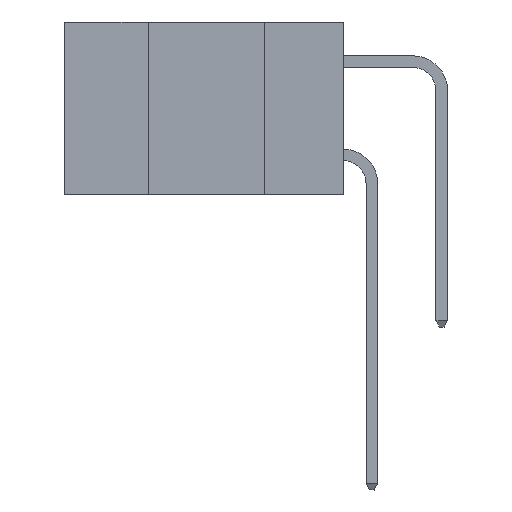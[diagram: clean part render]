
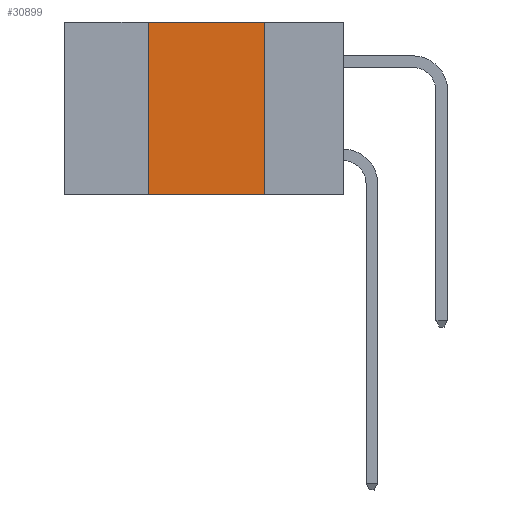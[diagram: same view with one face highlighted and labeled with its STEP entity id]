
A CAD part, left-side view. The second image highlights one B-rep face of the part: STEP entity #30899.
In plain terms, the highlighted planar face has unit normal (-1, 0, 0).
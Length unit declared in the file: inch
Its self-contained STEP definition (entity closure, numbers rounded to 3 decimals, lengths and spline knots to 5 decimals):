
#1603 = CARTESIAN_POINT ( 'NONE',  ( 0., 0.17, 0. ) ) ;
#2638 = LINE ( 'NONE', #18687, #22733 ) ;
#3861 = EDGE_LOOP ( 'NONE', ( #24879, #13345, #13877, #4963 ) ) ;
#4963 = ORIENTED_EDGE ( 'NONE', *, *, #8448, .T. ) ;
#5299 = VERTEX_POINT ( 'NONE', #20327 ) ;
#5952 = CARTESIAN_POINT ( 'NONE',  ( 0., 0.17, -0.37 ) ) ;
#6713 = AXIS2_PLACEMENT_3D ( 'NONE', #21900, #19490, #26617 ) ;
#8412 = DIRECTION ( 'NONE',  ( 0., -1., 0. ) ) ;
#8448 = EDGE_CURVE ( 'NONE', #5299, #20768, #2638, .T. ) ;
#8605 = DIRECTION ( 'NONE',  ( 0., 0., 1. ) ) ;
#9638 = FACE_OUTER_BOUND ( 'NONE', #3861, .T. ) ;
#12468 = VECTOR ( 'NONE', #21956, 39.37008 ) ;
#13230 = VERTEX_POINT ( 'NONE', #1603 ) ;
#13345 = ORIENTED_EDGE ( 'NONE', *, *, #16506, .F. ) ;
#13877 = ORIENTED_EDGE ( 'NONE', *, *, #30477, .F. ) ;
#14212 = EDGE_CURVE ( 'NONE', #13230, #20768, #14432, .T. ) ;
#14432 = LINE ( 'NONE', #19221, #12468 ) ;
#14481 = PLANE ( 'NONE',  #6713 ) ;
#15494 = VERTEX_POINT ( 'NONE', #31710 ) ;
#15525 = DIRECTION ( 'NONE',  ( 0., -1., 0. ) ) ;
#16506 = EDGE_CURVE ( 'NONE', #15494, #13230, #30037, .T. ) ;
#18687 = CARTESIAN_POINT ( 'NONE',  ( 0., 0.6, -0.37 ) ) ;
#18761 = CARTESIAN_POINT ( 'NONE',  ( 0., 0.42, 0. ) ) ;
#19221 = CARTESIAN_POINT ( 'NONE',  ( 0., 0.17, 0. ) ) ;
#19490 = DIRECTION ( 'NONE',  ( 1., 0., 0. ) ) ;
#20327 = CARTESIAN_POINT ( 'NONE',  ( 0., 0.42, -0.37 ) ) ;
#20768 = VERTEX_POINT ( 'NONE', #5952 ) ;
#21900 = CARTESIAN_POINT ( 'NONE',  ( 0., 0.6, 0. ) ) ;
#21907 = VECTOR ( 'NONE', #8605, 39.37008 ) ;
#21956 = DIRECTION ( 'NONE',  ( 0., 0., -1. ) ) ;
#22733 = VECTOR ( 'NONE', #8412, 39.37008 ) ;
#23373 = VECTOR ( 'NONE', #15525, 39.37008 ) ;
#24879 = ORIENTED_EDGE ( 'NONE', *, *, #14212, .F. ) ;
#25620 = CARTESIAN_POINT ( 'NONE',  ( 0., 0.6, 0. ) ) ;
#26617 = DIRECTION ( 'NONE',  ( 0., 0., -1. ) ) ;
#28559 = LINE ( 'NONE', #18761, #21907 ) ;
#30037 = LINE ( 'NONE', #25620, #23373 ) ;
#30477 = EDGE_CURVE ( 'NONE', #5299, #15494, #28559, .T. ) ;
#30899 = ADVANCED_FACE ( 'NONE', ( #9638 ), #14481, .F. ) ;
#31710 = CARTESIAN_POINT ( 'NONE',  ( 0., 0.42, 0. ) ) ;
